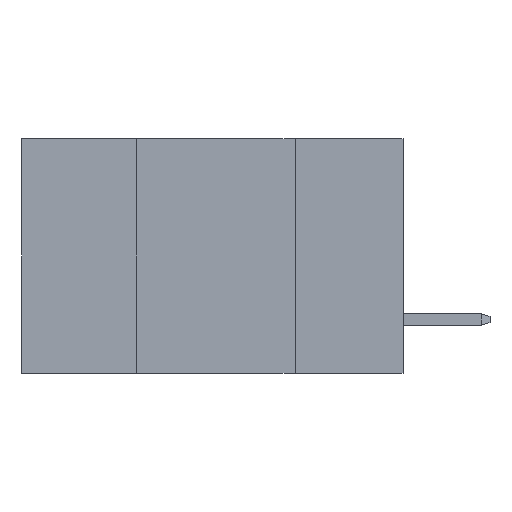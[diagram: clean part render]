
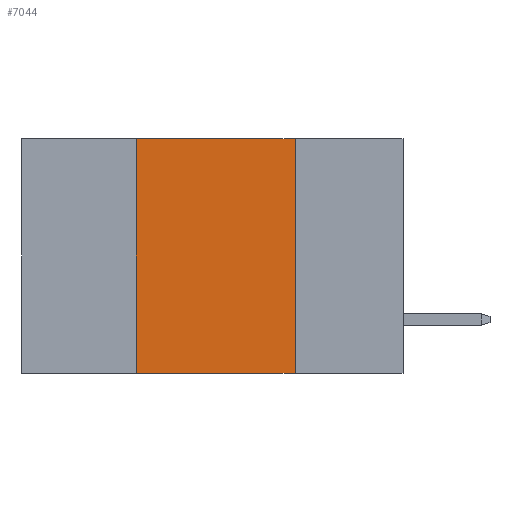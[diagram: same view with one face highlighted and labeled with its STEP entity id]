
A CAD part, left-side view. The second image highlights one B-rep face of the part: STEP entity #7044.
In plain terms, the highlighted planar face has unit normal (-1, 0, 0).
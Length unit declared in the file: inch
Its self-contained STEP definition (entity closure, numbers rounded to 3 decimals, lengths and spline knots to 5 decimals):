
#347 = CARTESIAN_POINT ( 'NONE',  ( 0., 0.6, 0. ) ) ;
#519 = VERTEX_POINT ( 'NONE', #5721 ) ;
#745 = CARTESIAN_POINT ( 'NONE',  ( 0., 0.17, 0. ) ) ;
#802 = DIRECTION ( 'NONE',  ( 0., -1., 0. ) ) ;
#923 = LINE ( 'NONE', #4559, #7849 ) ;
#1655 = DIRECTION ( 'NONE',  ( 0., 0., -1. ) ) ;
#2017 = ORIENTED_EDGE ( 'NONE', *, *, #7196, .F. ) ;
#3450 = ORIENTED_EDGE ( 'NONE', *, *, #9442, .F. ) ;
#3801 = VERTEX_POINT ( 'NONE', #7646 ) ;
#4559 = CARTESIAN_POINT ( 'NONE',  ( 0., 0.6, 0. ) ) ;
#4942 = LINE ( 'NONE', #8481, #10019 ) ;
#4945 = FACE_OUTER_BOUND ( 'NONE', #9947, .T. ) ;
#5106 = VERTEX_POINT ( 'NONE', #745 ) ;
#5721 = CARTESIAN_POINT ( 'NONE',  ( 0., 0.17, -0.37 ) ) ;
#7009 = VERTEX_POINT ( 'NONE', #10659 ) ;
#7044 = ADVANCED_FACE ( 'NONE', ( #4945 ), #8655, .F. ) ;
#7196 = EDGE_CURVE ( 'NONE', #3801, #7009, #9374, .T. ) ;
#7423 = VECTOR ( 'NONE', #8469, 39.37008 ) ;
#7646 = CARTESIAN_POINT ( 'NONE',  ( 0., 0.42, -0.37 ) ) ;
#7735 = DIRECTION ( 'NONE',  ( 1., 0., 0. ) ) ;
#7849 = VECTOR ( 'NONE', #802, 39.37008 ) ;
#7961 = ORIENTED_EDGE ( 'NONE', *, *, #10663, .T. ) ;
#8081 = LINE ( 'NONE', #11795, #9808 ) ;
#8469 = DIRECTION ( 'NONE',  ( 0., 0., 1. ) ) ;
#8481 = CARTESIAN_POINT ( 'NONE',  ( 0., 0.6, -0.37 ) ) ;
#8655 = PLANE ( 'NONE',  #9169 ) ;
#9169 = AXIS2_PLACEMENT_3D ( 'NONE', #347, #7735, #10537 ) ;
#9195 = CARTESIAN_POINT ( 'NONE',  ( 0., 0.42, 0. ) ) ;
#9374 = LINE ( 'NONE', #9195, #7423 ) ;
#9442 = EDGE_CURVE ( 'NONE', #7009, #5106, #923, .T. ) ;
#9808 = VECTOR ( 'NONE', #1655, 39.37008 ) ;
#9947 = EDGE_LOOP ( 'NONE', ( #11138, #3450, #2017, #7961 ) ) ;
#10019 = VECTOR ( 'NONE', #11202, 39.37008 ) ;
#10537 = DIRECTION ( 'NONE',  ( 0., 0., -1. ) ) ;
#10659 = CARTESIAN_POINT ( 'NONE',  ( 0., 0.42, 0. ) ) ;
#10663 = EDGE_CURVE ( 'NONE', #3801, #519, #4942, .T. ) ;
#11138 = ORIENTED_EDGE ( 'NONE', *, *, #11774, .F. ) ;
#11202 = DIRECTION ( 'NONE',  ( 0., -1., 0. ) ) ;
#11774 = EDGE_CURVE ( 'NONE', #5106, #519, #8081, .T. ) ;
#11795 = CARTESIAN_POINT ( 'NONE',  ( 0., 0.17, 0. ) ) ;
